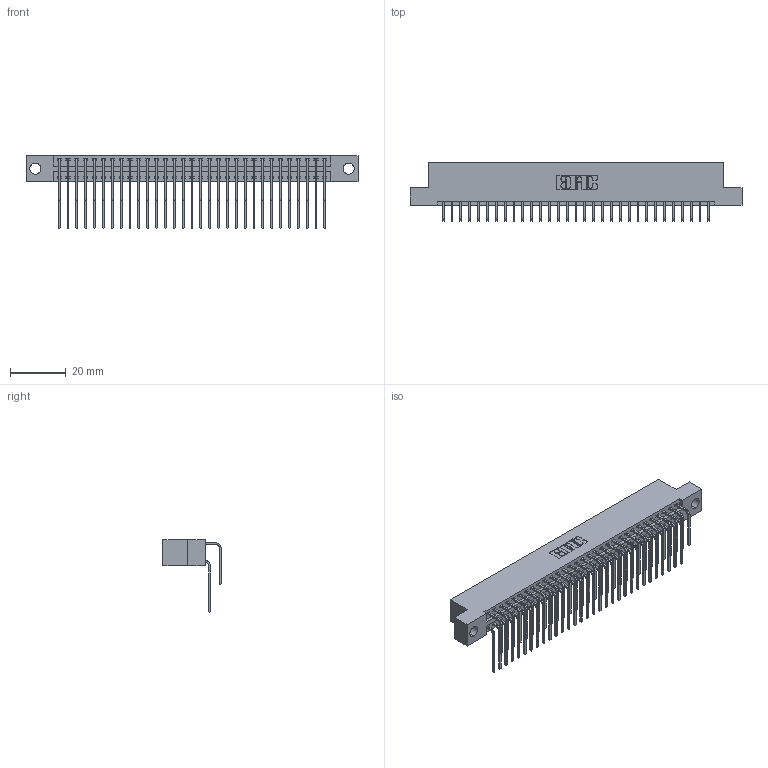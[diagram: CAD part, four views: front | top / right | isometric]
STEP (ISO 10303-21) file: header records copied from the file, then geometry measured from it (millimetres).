
FILE_DESCRIPTION (( 'STEP AP203' ), '1' );
FILE_NAME ('346-062-559-204.STEP', '2022-05-24T14:26:15', ( '' ), ( '' ), 'SwSTEP 2.0', 'SolidWorks 2020', '' );
FILE_SCHEMA (( 'CONFIG_CONTROL_DESIGN' ));
Length unit declared in the file: inch
Products named in the file (4): 346-062-559-204; 346 Part_Flush Mounting Lugs - 0.156 Dia-TH; 345-292-001_559 Tail - 2; 345-292-001_558 559 Tail - 1
Assembly tree (63 placements, depth 2):
  346-062-559-204
    346 Part_Flush Mounting Lugs - 0.156 Dia-TH
    345-292-001_558 559 Tail - 1  x31
    345-292-001_559 Tail - 2  x31
Bounding box: 119 x 20.89 x 26.16 mm (x, y, z)
Volume: 11770.2 mm3; surface area: 17569.7 mm2
Topology: 63 solids, 63 shells, 3484 faces, 10347 edges, 6814 vertices
Faces by surface type: plane 2384, cylinder 1100
Entity records: 23915 total; most frequent: CARTESIAN_POINT 4013, ORIENTED_EDGE 3894, DIRECTION 3559, EDGE_CURVE 1947, LINE 1651, VECTOR 1651, VERTEX_POINT 1294, AXIS2_PLACEMENT_3D 954
